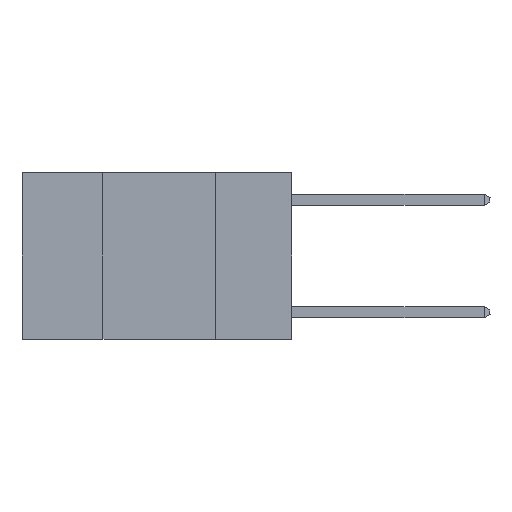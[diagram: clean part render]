
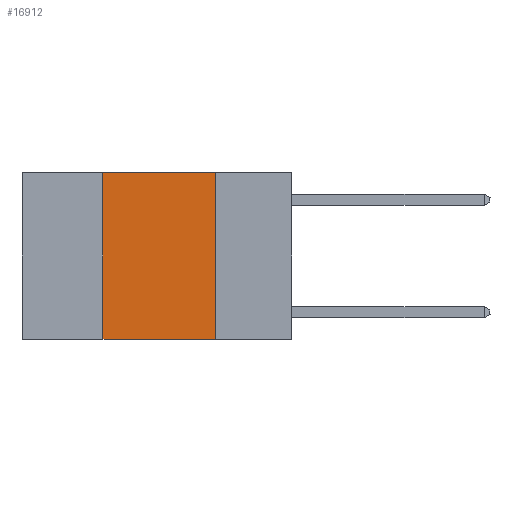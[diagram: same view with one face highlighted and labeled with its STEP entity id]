
A CAD part, left-side view. The second image highlights one B-rep face of the part: STEP entity #16912.
In plain terms, the highlighted planar face has unit normal (-1, 0, 0).
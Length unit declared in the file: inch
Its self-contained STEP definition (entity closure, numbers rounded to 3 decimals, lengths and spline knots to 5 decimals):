
#6 = ORIENTED_EDGE ( 'NONE', *, *, #12299, .F. ) ;
#2490 = DIRECTION ( 'NONE',  ( 1., 0., 0. ) ) ;
#3197 = CARTESIAN_POINT ( 'NONE',  ( 0., 0.17, 0. ) ) ;
#3815 = CARTESIAN_POINT ( 'NONE',  ( 0., 0.6, 0. ) ) ;
#3977 = EDGE_CURVE ( 'NONE', #17948, #15282, #19035, .T. ) ;
#4593 = ORIENTED_EDGE ( 'NONE', *, *, #3977, .F. ) ;
#5262 = LINE ( 'NONE', #3815, #6040 ) ;
#5323 = EDGE_CURVE ( 'NONE', #14666, #15282, #9006, .T. ) ;
#5598 = FACE_OUTER_BOUND ( 'NONE', #15140, .T. ) ;
#6011 = DIRECTION ( 'NONE',  ( 0., 0., -1. ) ) ;
#6040 = VECTOR ( 'NONE', #17310, 39.37008 ) ;
#6053 = CARTESIAN_POINT ( 'NONE',  ( 0., 0.42, 0. ) ) ;
#6098 = DIRECTION ( 'NONE',  ( 0., -1., 0. ) ) ;
#6589 = VECTOR ( 'NONE', #6011, 39.37008 ) ;
#7209 = LINE ( 'NONE', #6053, #10159 ) ;
#7921 = EDGE_CURVE ( 'NONE', #11344, #17948, #5262, .T. ) ;
#8823 = CARTESIAN_POINT ( 'NONE',  ( 0., 0.42, 0. ) ) ;
#9006 = LINE ( 'NONE', #11733, #16211 ) ;
#9059 = DIRECTION ( 'NONE',  ( 0., 0., 1. ) ) ;
#9267 = ORIENTED_EDGE ( 'NONE', *, *, #7921, .F. ) ;
#10152 = PLANE ( 'NONE',  #16820 ) ;
#10159 = VECTOR ( 'NONE', #9059, 39.37008 ) ;
#11344 = VERTEX_POINT ( 'NONE', #8823 ) ;
#11733 = CARTESIAN_POINT ( 'NONE',  ( 0., 0.6, -0.37 ) ) ;
#12299 = EDGE_CURVE ( 'NONE', #14666, #11344, #7209, .T. ) ;
#12517 = CARTESIAN_POINT ( 'NONE',  ( 0., 0.17, 0. ) ) ;
#13687 = CARTESIAN_POINT ( 'NONE',  ( 0., 0.17, -0.37 ) ) ;
#14393 = CARTESIAN_POINT ( 'NONE',  ( 0., 0.42, -0.37 ) ) ;
#14666 = VERTEX_POINT ( 'NONE', #14393 ) ;
#15140 = EDGE_LOOP ( 'NONE', ( #4593, #9267, #6, #16466 ) ) ;
#15282 = VERTEX_POINT ( 'NONE', #13687 ) ;
#16211 = VECTOR ( 'NONE', #6098, 39.37008 ) ;
#16466 = ORIENTED_EDGE ( 'NONE', *, *, #5323, .T. ) ;
#16820 = AXIS2_PLACEMENT_3D ( 'NONE', #18734, #2490, #17648 ) ;
#16912 = ADVANCED_FACE ( 'NONE', ( #5598 ), #10152, .F. ) ;
#17310 = DIRECTION ( 'NONE',  ( 0., -1., 0. ) ) ;
#17648 = DIRECTION ( 'NONE',  ( 0., 0., -1. ) ) ;
#17948 = VERTEX_POINT ( 'NONE', #12517 ) ;
#18734 = CARTESIAN_POINT ( 'NONE',  ( 0., 0.6, 0. ) ) ;
#19035 = LINE ( 'NONE', #3197, #6589 ) ;
